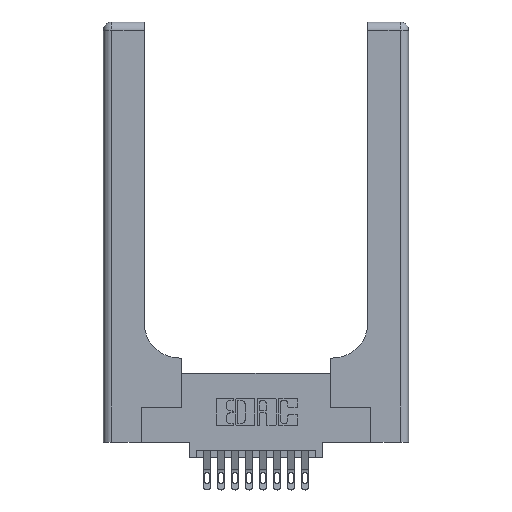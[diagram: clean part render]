
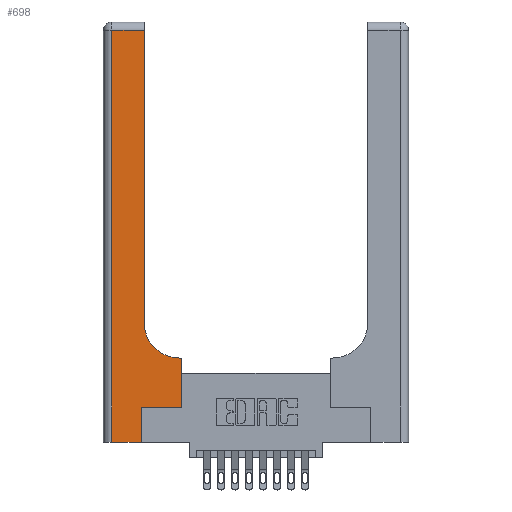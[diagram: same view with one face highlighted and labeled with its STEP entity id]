
A CAD part, top view. The second image highlights one B-rep face of the part: STEP entity #698.
In plain terms, the highlighted planar face has unit normal (0, 0, 1).
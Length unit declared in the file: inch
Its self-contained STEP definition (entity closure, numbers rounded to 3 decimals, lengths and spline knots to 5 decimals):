
#102 = CARTESIAN_POINT ( 'NONE',  ( 0.5415, 0.85, 0.37 ) ) ;
#205 = ORIENTED_EDGE ( 'NONE', *, *, #3569, .T. ) ;
#227 = EDGE_CURVE ( 'NONE', #5655, #4354, #12576, .T. ) ;
#354 = CARTESIAN_POINT ( 'NONE',  ( 0.2915, 0.6, 0.37 ) ) ;
#391 = DIRECTION ( 'NONE',  ( -1., 0., 0. ) ) ;
#698 = ADVANCED_FACE ( 'NONE', ( #10229 ), #5664, .F. ) ;
#946 = CARTESIAN_POINT ( 'NONE',  ( 0.269, 0.25, 0.37 ) ) ;
#1825 = EDGE_LOOP ( 'NONE', ( #3477, #14695, #5119, #7371, #4540, #3206, #3973, #15397, #205 ) ) ;
#1854 = CARTESIAN_POINT ( 'NONE',  ( 0.2915, 3., 0.37 ) ) ;
#2741 = CARTESIAN_POINT ( 'NONE',  ( 0.269, 0.25, 0.37 ) ) ;
#2790 = CARTESIAN_POINT ( 'NONE',  ( 0., 3., 0.37 ) ) ;
#2832 = DIRECTION ( 'NONE',  ( 1., 0., 0. ) ) ;
#2880 = DIRECTION ( 'NONE',  ( 0., 0., -1. ) ) ;
#3024 = AXIS2_PLACEMENT_3D ( 'NONE', #2790, #2880, #3182 ) ;
#3182 = DIRECTION ( 'NONE',  ( -1., 0., 0. ) ) ;
#3206 = ORIENTED_EDGE ( 'NONE', *, *, #3997, .T. ) ;
#3207 = CARTESIAN_POINT ( 'NONE',  ( 0.2915, 2.94, 0.37 ) ) ;
#3477 = ORIENTED_EDGE ( 'NONE', *, *, #5926, .T. ) ;
#3569 = EDGE_CURVE ( 'NONE', #9565, #7053, #9314, .T. ) ;
#3582 = CARTESIAN_POINT ( 'NONE',  ( 0.5415, 0.6, 0.37 ) ) ;
#3879 = AXIS2_PLACEMENT_3D ( 'NONE', #102, #11026, #16498 ) ;
#3931 = LINE ( 'NONE', #1854, #13765 ) ;
#3973 = ORIENTED_EDGE ( 'NONE', *, *, #4281, .T. ) ;
#3997 = EDGE_CURVE ( 'NONE', #9535, #15548, #5391, .T. ) ;
#4072 = EDGE_CURVE ( 'NONE', #6600, #9565, #8053, .T. ) ;
#4281 = EDGE_CURVE ( 'NONE', #15548, #6600, #12087, .T. ) ;
#4354 = VERTEX_POINT ( 'NONE', #4745 ) ;
#4540 = ORIENTED_EDGE ( 'NONE', *, *, #16191, .T. ) ;
#4572 = CARTESIAN_POINT ( 'NONE',  ( 0.5585, 0.25, 0.37 ) ) ;
#4745 = CARTESIAN_POINT ( 'NONE',  ( 0.06, 0., 0.37 ) ) ;
#4819 = EDGE_CURVE ( 'NONE', #4354, #5195, #14554, .T. ) ;
#5119 = ORIENTED_EDGE ( 'NONE', *, *, #227, .T. ) ;
#5195 = VERTEX_POINT ( 'NONE', #10604 ) ;
#5391 = LINE ( 'NONE', #2741, #8896 ) ;
#5655 = VERTEX_POINT ( 'NONE', #12762 ) ;
#5664 = PLANE ( 'NONE',  #3024 ) ;
#5926 = EDGE_CURVE ( 'NONE', #7053, #9362, #3931, .T. ) ;
#6330 = CARTESIAN_POINT ( 'NONE',  ( 0., 2.94, 0.37 ) ) ;
#6600 = VERTEX_POINT ( 'NONE', #12145 ) ;
#6660 = LINE ( 'NONE', #14457, #13052 ) ;
#7053 = VERTEX_POINT ( 'NONE', #14869 ) ;
#7371 = ORIENTED_EDGE ( 'NONE', *, *, #4819, .T. ) ;
#7723 = DIRECTION ( 'NONE',  ( -1., 0., 0. ) ) ;
#8053 = LINE ( 'NONE', #354, #14388 ) ;
#8671 = VECTOR ( 'NONE', #14751, 39.37008 ) ;
#8896 = VECTOR ( 'NONE', #2832, 39.37008 ) ;
#8966 = DIRECTION ( 'NONE',  ( 0., -1., 0. ) ) ;
#9001 = CARTESIAN_POINT ( 'NONE',  ( 0.06, 3., 0.37 ) ) ;
#9314 = CIRCLE ( 'NONE', #3879, 0.25 ) ;
#9362 = VERTEX_POINT ( 'NONE', #3207 ) ;
#9535 = VERTEX_POINT ( 'NONE', #946 ) ;
#9565 = VERTEX_POINT ( 'NONE', #3582 ) ;
#10229 = FACE_OUTER_BOUND ( 'NONE', #1825, .T. ) ;
#10604 = CARTESIAN_POINT ( 'NONE',  ( 0.269, 0., 0.37 ) ) ;
#11026 = DIRECTION ( 'NONE',  ( 0., 0., -1. ) ) ;
#11310 = VECTOR ( 'NONE', #13374, 39.37008 ) ;
#12087 = LINE ( 'NONE', #4572, #8671 ) ;
#12145 = CARTESIAN_POINT ( 'NONE',  ( 0.5585, 0.6, 0.37 ) ) ;
#12281 = VECTOR ( 'NONE', #7723, 39.37008 ) ;
#12576 = LINE ( 'NONE', #9001, #13313 ) ;
#12762 = CARTESIAN_POINT ( 'NONE',  ( 0.06, 2.94, 0.37 ) ) ;
#13052 = VECTOR ( 'NONE', #13213, 39.37008 ) ;
#13213 = DIRECTION ( 'NONE',  ( 0., 1., 0. ) ) ;
#13313 = VECTOR ( 'NONE', #8966, 39.37008 ) ;
#13374 = DIRECTION ( 'NONE',  ( 1., 0., 0. ) ) ;
#13765 = VECTOR ( 'NONE', #15787, 39.37008 ) ;
#14149 = CARTESIAN_POINT ( 'NONE',  ( 0.5585, 0.25, 0.37 ) ) ;
#14388 = VECTOR ( 'NONE', #391, 39.37008 ) ;
#14457 = CARTESIAN_POINT ( 'NONE',  ( 0.269, 0., 0.37 ) ) ;
#14554 = LINE ( 'NONE', #15772, #11310 ) ;
#14695 = ORIENTED_EDGE ( 'NONE', *, *, #16031, .T. ) ;
#14751 = DIRECTION ( 'NONE',  ( 0., 1., 0. ) ) ;
#14869 = CARTESIAN_POINT ( 'NONE',  ( 0.2915, 0.85, 0.37 ) ) ;
#15009 = LINE ( 'NONE', #6330, #12281 ) ;
#15397 = ORIENTED_EDGE ( 'NONE', *, *, #4072, .T. ) ;
#15548 = VERTEX_POINT ( 'NONE', #14149 ) ;
#15772 = CARTESIAN_POINT ( 'NONE',  ( 0., 0., 0.37 ) ) ;
#15787 = DIRECTION ( 'NONE',  ( 0., 1., 0. ) ) ;
#16031 = EDGE_CURVE ( 'NONE', #9362, #5655, #15009, .T. ) ;
#16191 = EDGE_CURVE ( 'NONE', #5195, #9535, #6660, .T. ) ;
#16498 = DIRECTION ( 'NONE',  ( 1., 0., 0. ) ) ;
